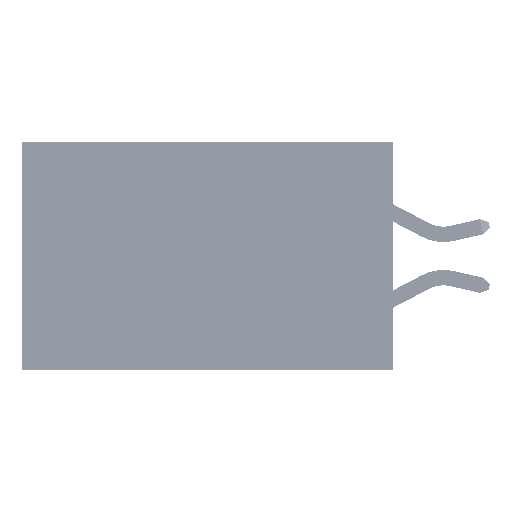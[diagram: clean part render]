
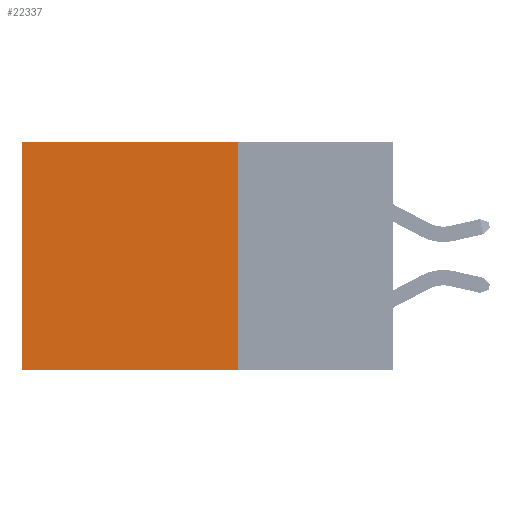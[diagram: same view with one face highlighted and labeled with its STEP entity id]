
A CAD part, left-side view. The second image highlights one B-rep face of the part: STEP entity #22337.
In plain terms, the highlighted planar face has unit normal (-1, 0, 0).
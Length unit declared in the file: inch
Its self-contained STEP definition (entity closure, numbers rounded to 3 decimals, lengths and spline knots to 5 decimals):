
#1784 = ORIENTED_EDGE ( 'NONE', *, *, #27185, .T. ) ;
#5166 = VECTOR ( 'NONE', #33244, 39.37008 ) ;
#6393 = VERTEX_POINT ( 'NONE', #13452 ) ;
#6413 = DIRECTION ( 'NONE',  ( 1., 0., 0. ) ) ;
#7919 = AXIS2_PLACEMENT_3D ( 'NONE', #34152, #6413, #50024 ) ;
#8766 = FACE_OUTER_BOUND ( 'NONE', #33913, .T. ) ;
#10539 = CARTESIAN_POINT ( 'NONE',  ( 0.2875, 0.25, 0. ) ) ;
#12396 = VECTOR ( 'NONE', #17813, 39.37008 ) ;
#13452 = CARTESIAN_POINT ( 'NONE',  ( 0.2875, 0.25, 0. ) ) ;
#14039 = EDGE_CURVE ( 'NONE', #6393, #30993, #34706, .T. ) ;
#17813 = DIRECTION ( 'NONE',  ( 0., 0., -1. ) ) ;
#18831 = ORIENTED_EDGE ( 'NONE', *, *, #44486, .F. ) ;
#21886 = VERTEX_POINT ( 'NONE', #35353 ) ;
#22337 = ADVANCED_FACE ( 'NONE', ( #8766 ), #26049, .F. ) ;
#23533 = CARTESIAN_POINT ( 'NONE',  ( 0.2875, 0.6, 0. ) ) ;
#23541 = VECTOR ( 'NONE', #42873, 39.37008 ) ;
#26049 = PLANE ( 'NONE',  #7919 ) ;
#26307 = LINE ( 'NONE', #10539, #5166 ) ;
#27185 = EDGE_CURVE ( 'NONE', #45401, #21886, #38367, .T. ) ;
#30342 = ORIENTED_EDGE ( 'NONE', *, *, #14039, .F. ) ;
#30993 = VERTEX_POINT ( 'NONE', #40931 ) ;
#32524 = LINE ( 'NONE', #50991, #33114 ) ;
#33114 = VECTOR ( 'NONE', #39086, 39.37008 ) ;
#33244 = DIRECTION ( 'NONE',  ( 0., 1., 0. ) ) ;
#33482 = EDGE_CURVE ( 'NONE', #6393, #45401, #26307, .T. ) ;
#33913 = EDGE_LOOP ( 'NONE', ( #1784, #18831, #30342, #43744 ) ) ;
#34152 = CARTESIAN_POINT ( 'NONE',  ( 0.2875, 0.25, 0. ) ) ;
#34706 = LINE ( 'NONE', #37380, #12396 ) ;
#35353 = CARTESIAN_POINT ( 'NONE',  ( 0.2875, 0.6, -0.37 ) ) ;
#37380 = CARTESIAN_POINT ( 'NONE',  ( 0.2875, 0.25, 0. ) ) ;
#38367 = LINE ( 'NONE', #23533, #23541 ) ;
#39086 = DIRECTION ( 'NONE',  ( 0., 1., 0. ) ) ;
#40931 = CARTESIAN_POINT ( 'NONE',  ( 0.2875, 0.25, -0.37 ) ) ;
#42873 = DIRECTION ( 'NONE',  ( 0., 0., -1. ) ) ;
#43744 = ORIENTED_EDGE ( 'NONE', *, *, #33482, .T. ) ;
#44486 = EDGE_CURVE ( 'NONE', #30993, #21886, #32524, .T. ) ;
#45401 = VERTEX_POINT ( 'NONE', #50298 ) ;
#50024 = DIRECTION ( 'NONE',  ( 0., 0., -1. ) ) ;
#50298 = CARTESIAN_POINT ( 'NONE',  ( 0.2875, 0.6, 0. ) ) ;
#50991 = CARTESIAN_POINT ( 'NONE',  ( 0.2875, 0.25, -0.37 ) ) ;
